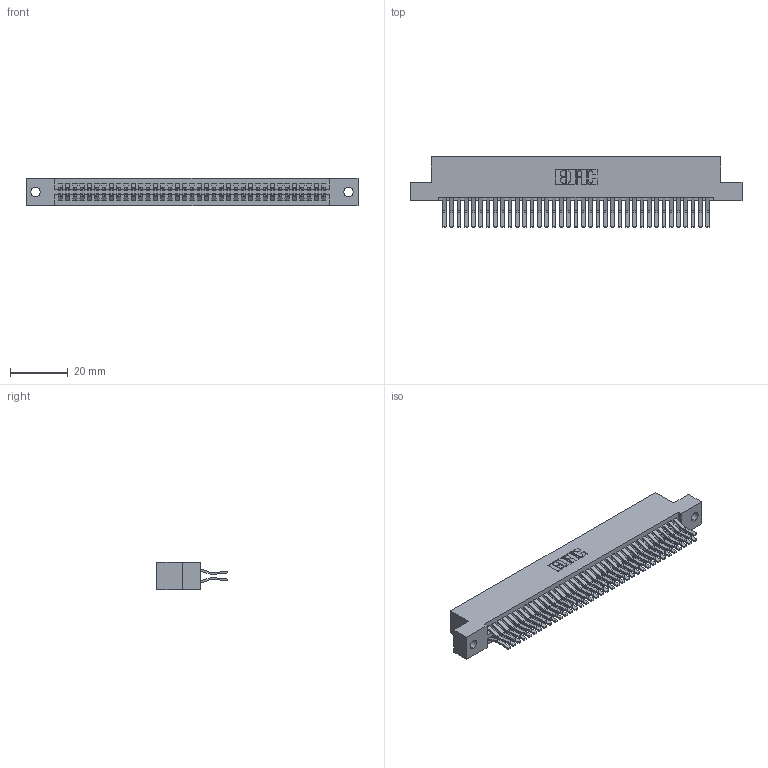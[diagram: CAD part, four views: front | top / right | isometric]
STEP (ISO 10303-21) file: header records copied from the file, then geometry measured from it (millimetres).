
FILE_DESCRIPTION (( 'STEP AP203' ), '1' );
FILE_NAME ('345-074-560-202.STEP', '2018-10-02T14:21:07', ( '' ), ( '' ), 'SwSTEP 2.0', 'SolidWorks 2016', '' );
FILE_SCHEMA (( 'CONFIG_CONTROL_DESIGN' ));
Length unit declared in the file: inch
Products named in the file (3): 345-074-560-202; 345-292-001_560 Tail; 345 Part_Flush Mounting Lugs - 0.128 Dia
Assembly tree (75 placements, depth 2):
  345-074-560-202
    345 Part_Flush Mounting Lugs - 0.128 Dia
    345-292-001_560 Tail  x74
Bounding box: 115.19 x 24.45 x 9.4 mm (x, y, z)
Volume: 11591.5 mm3; surface area: 18012.1 mm2
Topology: 75 solids, 75 shells, 3974 faces, 11811 edges, 7774 vertices
Faces by surface type: plane 2522, cylinder 1452
Entity records: 29795 total; most frequent: CARTESIAN_POINT 5000, ORIENTED_EDGE 4934, DIRECTION 4419, EDGE_CURVE 2467, VECTOR 2183, LINE 2183, VERTEX_POINT 1642, AXIS2_PLACEMENT_3D 1118
